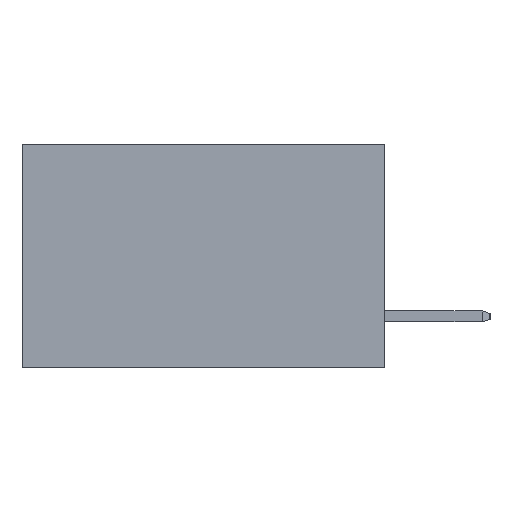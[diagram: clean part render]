
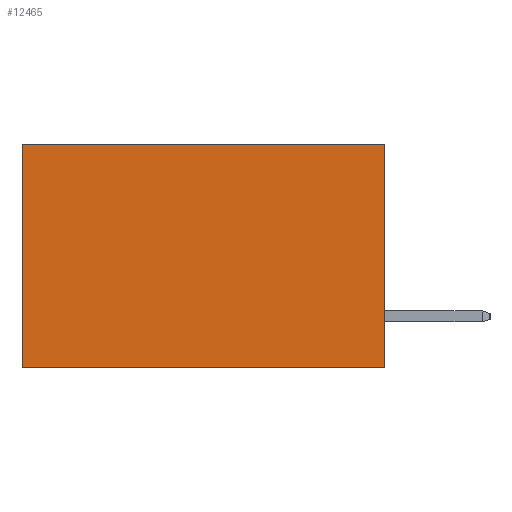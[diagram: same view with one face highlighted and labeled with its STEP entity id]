
A CAD part, left-side view. The second image highlights one B-rep face of the part: STEP entity #12465.
In plain terms, the highlighted planar face has unit normal (-1, 0, 0).
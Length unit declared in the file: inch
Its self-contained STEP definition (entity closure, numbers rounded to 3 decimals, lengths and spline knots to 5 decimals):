
#443 = CARTESIAN_POINT ( 'NONE',  ( 0.2615, 0.6, 0. ) ) ;
#477 = ORIENTED_EDGE ( 'NONE', *, *, #14193, .F. ) ;
#1115 = VECTOR ( 'NONE', #10965, 39.37008 ) ;
#1143 = LINE ( 'NONE', #12182, #12627 ) ;
#2338 = VERTEX_POINT ( 'NONE', #12509 ) ;
#3123 = DIRECTION ( 'NONE',  ( 1., 0., 0. ) ) ;
#3884 = ORIENTED_EDGE ( 'NONE', *, *, #5416, .T. ) ;
#3967 = DIRECTION ( 'NONE',  ( 0., 1., 0. ) ) ;
#4921 = FACE_OUTER_BOUND ( 'NONE', #12326, .T. ) ;
#5287 = VECTOR ( 'NONE', #14345, 39.37008 ) ;
#5416 = EDGE_CURVE ( 'NONE', #12273, #2338, #1143, .T. ) ;
#6738 = VERTEX_POINT ( 'NONE', #12387 ) ;
#7291 = AXIS2_PLACEMENT_3D ( 'NONE', #12287, #3123, #11176 ) ;
#7457 = CARTESIAN_POINT ( 'NONE',  ( 0.2615, 0., -0.37 ) ) ;
#7725 = PLANE ( 'NONE',  #7291 ) ;
#7956 = CARTESIAN_POINT ( 'NONE',  ( 0.2615, 0., 0. ) ) ;
#9102 = LINE ( 'NONE', #9717, #12838 ) ;
#9717 = CARTESIAN_POINT ( 'NONE',  ( 0.2615, 0., 0. ) ) ;
#9755 = EDGE_CURVE ( 'NONE', #14433, #12273, #9102, .T. ) ;
#10533 = ORIENTED_EDGE ( 'NONE', *, *, #12851, .F. ) ;
#10965 = DIRECTION ( 'NONE',  ( 0., 0., -1. ) ) ;
#11176 = DIRECTION ( 'NONE',  ( 0., 0., -1. ) ) ;
#12182 = CARTESIAN_POINT ( 'NONE',  ( 0.2615, 0.6, -0.37 ) ) ;
#12273 = VERTEX_POINT ( 'NONE', #443 ) ;
#12287 = CARTESIAN_POINT ( 'NONE',  ( 0.2615, 0., -0.37 ) ) ;
#12326 = EDGE_LOOP ( 'NONE', ( #3884, #10533, #477, #14112 ) ) ;
#12387 = CARTESIAN_POINT ( 'NONE',  ( 0.2615, 0., -0.37 ) ) ;
#12465 = ADVANCED_FACE ( 'NONE', ( #4921 ), #7725, .F. ) ;
#12509 = CARTESIAN_POINT ( 'NONE',  ( 0.2615, 0.6, -0.37 ) ) ;
#12627 = VECTOR ( 'NONE', #13388, 39.37008 ) ;
#12838 = VECTOR ( 'NONE', #3967, 39.37008 ) ;
#12851 = EDGE_CURVE ( 'NONE', #6738, #2338, #14799, .T. ) ;
#13321 = LINE ( 'NONE', #14385, #1115 ) ;
#13388 = DIRECTION ( 'NONE',  ( 0., 0., -1. ) ) ;
#14112 = ORIENTED_EDGE ( 'NONE', *, *, #9755, .T. ) ;
#14193 = EDGE_CURVE ( 'NONE', #14433, #6738, #13321, .T. ) ;
#14345 = DIRECTION ( 'NONE',  ( 0., 1., 0. ) ) ;
#14385 = CARTESIAN_POINT ( 'NONE',  ( 0.2615, 0., -0.37 ) ) ;
#14433 = VERTEX_POINT ( 'NONE', #7956 ) ;
#14799 = LINE ( 'NONE', #7457, #5287 ) ;
